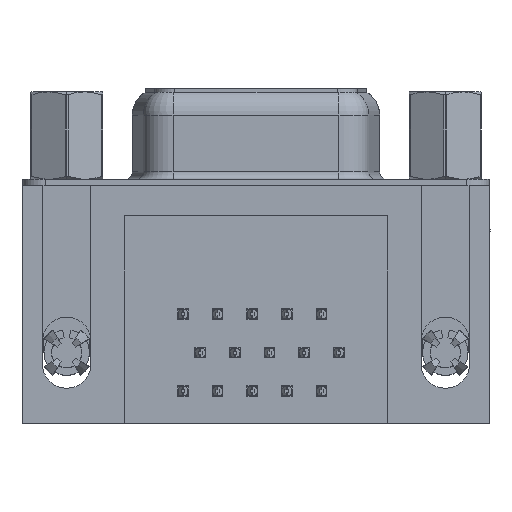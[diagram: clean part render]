
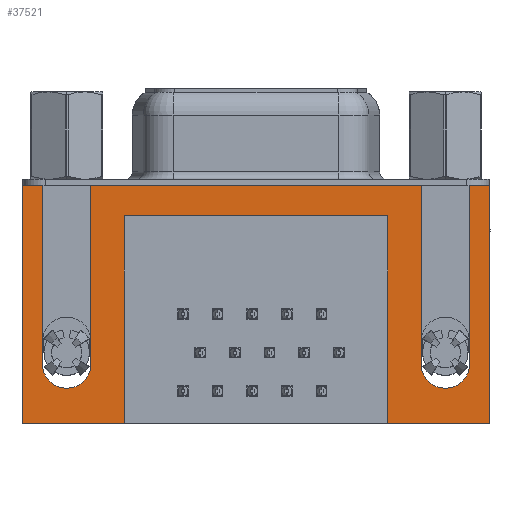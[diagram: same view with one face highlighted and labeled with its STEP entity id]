
A CAD part, front view. The second image highlights one B-rep face of the part: STEP entity #37521.
In plain terms, the highlighted planar face has unit normal (0, -1, 0).
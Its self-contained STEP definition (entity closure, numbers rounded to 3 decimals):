
#243 = DIRECTION ( 'NONE',  ( 0., 0., 1. ) ) ;
#389 = CARTESIAN_POINT ( 'NONE',  ( 26.59, -6.275, 0. ) ) ;
#697 = DIRECTION ( 'NONE',  ( 0., -1., 0. ) ) ;
#1756 = EDGE_CURVE ( 'NONE', #23516, #40730, #18913, .T. ) ;
#2353 = CARTESIAN_POINT ( 'NONE',  ( 27.9, -6.275, 0. ) ) ;
#3193 = ORIENTED_EDGE ( 'NONE', *, *, #6506, .F. ) ;
#3287 = VERTEX_POINT ( 'NONE', #42300 ) ;
#3830 = ORIENTED_EDGE ( 'NONE', *, *, #8274, .F. ) ;
#4425 = LINE ( 'NONE', #39926, #4884 ) ;
#4474 = LINE ( 'NONE', #19469, #14356 ) ;
#4508 = LINE ( 'NONE', #42397, #21336 ) ;
#4719 = VERTEX_POINT ( 'NONE', #31893 ) ;
#4884 = VECTOR ( 'NONE', #43283, 1000. ) ;
#5514 = EDGE_CURVE ( 'NONE', #16455, #28548, #43001, .T. ) ;
#6001 = CARTESIAN_POINT ( 'NONE',  ( 26.59, -6.275, 0. ) ) ;
#6506 = EDGE_CURVE ( 'NONE', #28548, #3287, #25242, .T. ) ;
#7177 = ORIENTED_EDGE ( 'NONE', *, *, #39129, .F. ) ;
#7235 = EDGE_CURVE ( 'NONE', #3287, #19638, #42611, .T. ) ;
#7285 = CARTESIAN_POINT ( 'NONE',  ( -2.91, -6.275, 0. ) ) ;
#7346 = ORIENTED_EDGE ( 'NONE', *, *, #8079, .F. ) ;
#7429 = EDGE_CURVE ( 'NONE', #19638, #39881, #41865, .T. ) ;
#7822 = EDGE_CURVE ( 'NONE', #39881, #16241, #36982, .T. ) ;
#8079 = EDGE_CURVE ( 'NONE', #19066, #16999, #34736, .T. ) ;
#8274 = EDGE_CURVE ( 'NONE', #4719, #29558, #33260, .T. ) ;
#8532 = LINE ( 'NONE', #12112, #24303 ) ;
#8625 = EDGE_CURVE ( 'NONE', #9480, #23516, #31344, .T. ) ;
#8858 = EDGE_CURVE ( 'NONE', #40730, #38054, #29037, .T. ) ;
#9142 = DIRECTION ( 'NONE',  ( 0., 0., -1. ) ) ;
#9480 = VERTEX_POINT ( 'NONE', #39328 ) ;
#9587 = ORIENTED_EDGE ( 'NONE', *, *, #36454, .F. ) ;
#9665 = AXIS2_PLACEMENT_3D ( 'NONE', #12640, #30560, #34182 ) ;
#11004 = CARTESIAN_POINT ( 'NONE',  ( 1.6, -6.275, 0. ) ) ;
#11417 = CARTESIAN_POINT ( 'NONE',  ( 27.9, -6.275, -15.7 ) ) ;
#11597 = CARTESIAN_POINT ( 'NONE',  ( 27.9, -6.275, -15.7 ) ) ;
#11814 = CARTESIAN_POINT ( 'NONE',  ( -1.6, -6.275, -11.78 ) ) ;
#12112 = CARTESIAN_POINT ( 'NONE',  ( -2.91, -6.275, 0. ) ) ;
#12640 = CARTESIAN_POINT ( 'NONE',  ( 24.99, -6.275, -11.78 ) ) ;
#13020 = DIRECTION ( 'NONE',  ( -1., 0., 0. ) ) ;
#13069 = CARTESIAN_POINT ( 'NONE',  ( 27.9, -6.275, -15.7 ) ) ;
#13902 = CIRCLE ( 'NONE', #23748, 1.6 ) ;
#14356 = VECTOR ( 'NONE', #42928, 1000. ) ;
#14476 = CARTESIAN_POINT ( 'NONE',  ( 3.79, -6.275, -15.7 ) ) ;
#15208 = ORIENTED_EDGE ( 'NONE', *, *, #32650, .F. ) ;
#15681 = EDGE_CURVE ( 'NONE', #16455, #17143, #4425, .T. ) ;
#16070 = CARTESIAN_POINT ( 'NONE',  ( 3.79, -6.275, -2. ) ) ;
#16199 = VECTOR ( 'NONE', #40840, 1000. ) ;
#16241 = VERTEX_POINT ( 'NONE', #20095 ) ;
#16455 = VERTEX_POINT ( 'NONE', #11417 ) ;
#16999 = VERTEX_POINT ( 'NONE', #11814 ) ;
#17143 = VERTEX_POINT ( 'NONE', #2353 ) ;
#17576 = EDGE_LOOP ( 'NONE', ( #35171, #17963, #40921, #7177, #3830, #15208, #7346, #27379, #27278, #18305, #41377, #41527, #3193, #25153, #21503, #9587 ) ) ;
#17845 = CARTESIAN_POINT ( 'NONE',  ( 23.39, -6.275, -11.78 ) ) ;
#17963 = ORIENTED_EDGE ( 'NONE', *, *, #1756, .F. ) ;
#18305 = ORIENTED_EDGE ( 'NONE', *, *, #7822, .F. ) ;
#18428 = CARTESIAN_POINT ( 'NONE',  ( 21.2, -6.275, -2. ) ) ;
#18913 = CIRCLE ( 'NONE', #9665, 1.6 ) ;
#19066 = VERTEX_POINT ( 'NONE', #43482 ) ;
#19469 = CARTESIAN_POINT ( 'NONE',  ( -2.91, -6.275, 0. ) ) ;
#19638 = VERTEX_POINT ( 'NONE', #16070 ) ;
#19994 = EDGE_CURVE ( 'NONE', #16241, #23273, #4508, .T. ) ;
#20095 = CARTESIAN_POINT ( 'NONE',  ( -2.91, -6.275, -15.7 ) ) ;
#20492 = CARTESIAN_POINT ( 'NONE',  ( 1.6, -6.275, 0. ) ) ;
#20956 = CARTESIAN_POINT ( 'NONE',  ( 0., -6.275, -11.78 ) ) ;
#21336 = VECTOR ( 'NONE', #29063, 1000. ) ;
#21503 = ORIENTED_EDGE ( 'NONE', *, *, #15681, .T. ) ;
#23273 = VERTEX_POINT ( 'NONE', #30227 ) ;
#23399 = DIRECTION ( 'NONE',  ( 0., 0., -1. ) ) ;
#23516 = VERTEX_POINT ( 'NONE', #17845 ) ;
#23622 = CARTESIAN_POINT ( 'NONE',  ( 26.59, -6.275, -11.78 ) ) ;
#23748 = AXIS2_PLACEMENT_3D ( 'NONE', #20956, #697, #24360 ) ;
#24303 = VECTOR ( 'NONE', #32271, 1000. ) ;
#24360 = DIRECTION ( 'NONE',  ( 1., 0., 0. ) ) ;
#25153 = ORIENTED_EDGE ( 'NONE', *, *, #5514, .F. ) ;
#25234 = VECTOR ( 'NONE', #28618, 1000. ) ;
#25242 = LINE ( 'NONE', #18428, #25234 ) ;
#25897 = PLANE ( 'NONE',  #38749 ) ;
#25996 = CARTESIAN_POINT ( 'NONE',  ( 23.39, -6.275, 0. ) ) ;
#26502 = CARTESIAN_POINT ( 'NONE',  ( 3.79, -6.275, -2. ) ) ;
#27278 = ORIENTED_EDGE ( 'NONE', *, *, #19994, .F. ) ;
#27379 = ORIENTED_EDGE ( 'NONE', *, *, #39761, .F. ) ;
#28548 = VERTEX_POINT ( 'NONE', #31442 ) ;
#28618 = DIRECTION ( 'NONE',  ( 0., 0., 1. ) ) ;
#28820 = VECTOR ( 'NONE', #243, 1000. ) ;
#29037 = LINE ( 'NONE', #389, #28820 ) ;
#29063 = DIRECTION ( 'NONE',  ( 0., 0., 1. ) ) ;
#29221 = DIRECTION ( 'NONE',  ( 0., -1., 0. ) ) ;
#29558 = VERTEX_POINT ( 'NONE', #20492 ) ;
#29806 = DIRECTION ( 'NONE',  ( 0., 0., -1. ) ) ;
#30227 = CARTESIAN_POINT ( 'NONE',  ( -2.91, -6.275, 0. ) ) ;
#30560 = DIRECTION ( 'NONE',  ( 0., -1., 0. ) ) ;
#31344 = LINE ( 'NONE', #25996, #31637 ) ;
#31442 = CARTESIAN_POINT ( 'NONE',  ( 21.2, -6.275, -15.7 ) ) ;
#31637 = VECTOR ( 'NONE', #32705, 1000. ) ;
#31893 = CARTESIAN_POINT ( 'NONE',  ( 1.6, -6.275, -11.78 ) ) ;
#32069 = CARTESIAN_POINT ( 'NONE',  ( 3.79, -6.275, -2. ) ) ;
#32271 = DIRECTION ( 'NONE',  ( 1., 0., 0. ) ) ;
#32324 = CARTESIAN_POINT ( 'NONE',  ( -2.91, -6.275, -2.5 ) ) ;
#32650 = EDGE_CURVE ( 'NONE', #16999, #4719, #13902, .T. ) ;
#32705 = DIRECTION ( 'NONE',  ( 0., 0., -1. ) ) ;
#33218 = VECTOR ( 'NONE', #34540, 1000. ) ;
#33260 = LINE ( 'NONE', #11004, #33218 ) ;
#34182 = DIRECTION ( 'NONE',  ( -1., 0., 0. ) ) ;
#34540 = DIRECTION ( 'NONE',  ( 0., 0., 1. ) ) ;
#34736 = LINE ( 'NONE', #36857, #35120 ) ;
#35120 = VECTOR ( 'NONE', #23399, 1000. ) ;
#35171 = ORIENTED_EDGE ( 'NONE', *, *, #8858, .F. ) ;
#36317 = LINE ( 'NONE', #7285, #16199 ) ;
#36454 = EDGE_CURVE ( 'NONE', #38054, #17143, #4474, .T. ) ;
#36563 = VECTOR ( 'NONE', #38477, 1000. ) ;
#36857 = CARTESIAN_POINT ( 'NONE',  ( -1.6, -6.275, 0. ) ) ;
#36982 = LINE ( 'NONE', #11597, #36563 ) ;
#37521 = ADVANCED_FACE ( 'NONE', ( #39567 ), #25897, .T. ) ;
#38054 = VERTEX_POINT ( 'NONE', #6001 ) ;
#38477 = DIRECTION ( 'NONE',  ( -1., 0., 0. ) ) ;
#38749 = AXIS2_PLACEMENT_3D ( 'NONE', #32324, #29221, #9142 ) ;
#39129 = EDGE_CURVE ( 'NONE', #29558, #9480, #8532, .T. ) ;
#39328 = CARTESIAN_POINT ( 'NONE',  ( 23.39, -6.275, 0. ) ) ;
#39567 = FACE_OUTER_BOUND ( 'NONE', #17576, .T. ) ;
#39761 = EDGE_CURVE ( 'NONE', #23273, #19066, #36317, .T. ) ;
#39881 = VERTEX_POINT ( 'NONE', #14476 ) ;
#39926 = CARTESIAN_POINT ( 'NONE',  ( 27.9, -6.275, -2.5 ) ) ;
#40730 = VERTEX_POINT ( 'NONE', #23622 ) ;
#40840 = DIRECTION ( 'NONE',  ( 1., 0., 0. ) ) ;
#40921 = ORIENTED_EDGE ( 'NONE', *, *, #8625, .F. ) ;
#41368 = VECTOR ( 'NONE', #29806, 1000. ) ;
#41377 = ORIENTED_EDGE ( 'NONE', *, *, #7429, .F. ) ;
#41527 = ORIENTED_EDGE ( 'NONE', *, *, #7235, .F. ) ;
#41865 = LINE ( 'NONE', #26502, #41368 ) ;
#42155 = DIRECTION ( 'NONE',  ( -1., 0., 0. ) ) ;
#42300 = CARTESIAN_POINT ( 'NONE',  ( 21.2, -6.275, -2. ) ) ;
#42397 = CARTESIAN_POINT ( 'NONE',  ( -2.91, -6.275, -2.5 ) ) ;
#42555 = VECTOR ( 'NONE', #42155, 1000. ) ;
#42611 = LINE ( 'NONE', #32069, #42555 ) ;
#42924 = VECTOR ( 'NONE', #13020, 1000. ) ;
#42928 = DIRECTION ( 'NONE',  ( 1., 0., 0. ) ) ;
#43001 = LINE ( 'NONE', #13069, #42924 ) ;
#43283 = DIRECTION ( 'NONE',  ( 0., 0., 1. ) ) ;
#43482 = CARTESIAN_POINT ( 'NONE',  ( -1.6, -6.275, 0. ) ) ;
